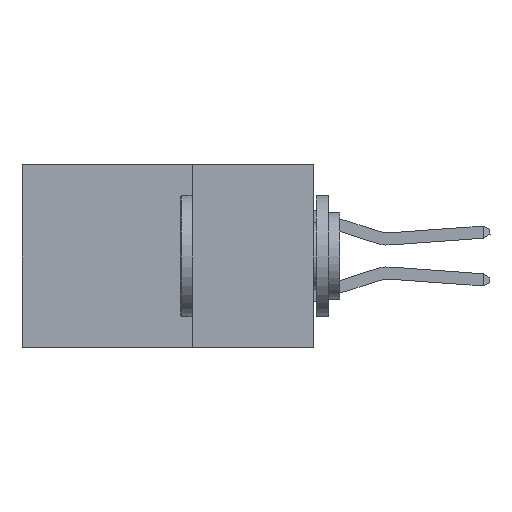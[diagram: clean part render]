
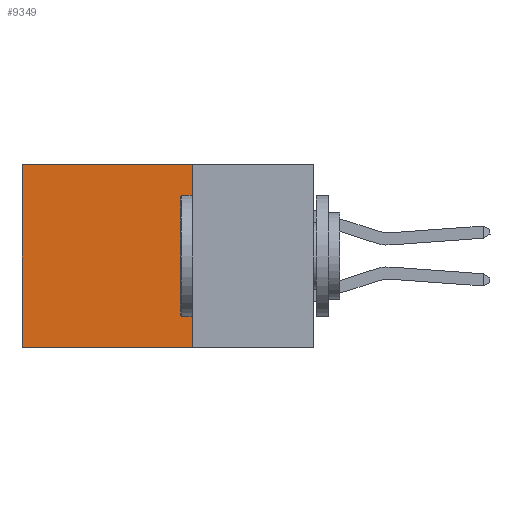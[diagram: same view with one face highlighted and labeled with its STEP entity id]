
A CAD part, left-side view. The second image highlights one B-rep face of the part: STEP entity #9349.
In plain terms, the highlighted planar face has unit normal (-1, 0, 0).
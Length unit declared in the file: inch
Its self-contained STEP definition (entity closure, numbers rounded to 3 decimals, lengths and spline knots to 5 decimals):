
#368 = VERTEX_POINT ( 'NONE', #6260 ) ;
#811 = DIRECTION ( 'NONE',  ( 0., 1., 0. ) ) ;
#1485 = CARTESIAN_POINT ( 'NONE',  ( 0.2875, 0.6, -0.375 ) ) ;
#2697 = AXIS2_PLACEMENT_3D ( 'NONE', #14191, #8348, #5224 ) ;
#2864 = VECTOR ( 'NONE', #811, 39.37008 ) ;
#2972 = ORIENTED_EDGE ( 'NONE', *, *, #7686, .F. ) ;
#3616 = CARTESIAN_POINT ( 'NONE',  ( 0.2875, 0.6, 0. ) ) ;
#3861 = DIRECTION ( 'NONE',  ( 0., 1., 0. ) ) ;
#5224 = DIRECTION ( 'NONE',  ( 0., 0., -1. ) ) ;
#5724 = CARTESIAN_POINT ( 'NONE',  ( 0.2875, 0.25, -0.375 ) ) ;
#6260 = CARTESIAN_POINT ( 'NONE',  ( 0.2875, 0.6, -0.375 ) ) ;
#6409 = CARTESIAN_POINT ( 'NONE',  ( 0.2875, 0.25, -0.375 ) ) ;
#7025 = EDGE_CURVE ( 'NONE', #10077, #368, #10886, .T. ) ;
#7678 = VERTEX_POINT ( 'NONE', #15529 ) ;
#7686 = EDGE_CURVE ( 'NONE', #7678, #10077, #18192, .T. ) ;
#8348 = DIRECTION ( 'NONE',  ( 1., 0., 0. ) ) ;
#9180 = VECTOR ( 'NONE', #10527, 39.37008 ) ;
#9344 = EDGE_CURVE ( 'NONE', #7678, #10639, #14052, .T. ) ;
#9349 = ADVANCED_FACE ( 'NONE', ( #13579 ), #19061, .F. ) ;
#9946 = EDGE_LOOP ( 'NONE', ( #19256, #12822, #2972, #17347 ) ) ;
#10061 = VECTOR ( 'NONE', #3861, 39.37008 ) ;
#10077 = VERTEX_POINT ( 'NONE', #5724 ) ;
#10527 = DIRECTION ( 'NONE',  ( 0., 0., -1. ) ) ;
#10639 = VERTEX_POINT ( 'NONE', #3616 ) ;
#10886 = LINE ( 'NONE', #14445, #2864 ) ;
#12457 = LINE ( 'NONE', #1485, #9180 ) ;
#12822 = ORIENTED_EDGE ( 'NONE', *, *, #7025, .F. ) ;
#13579 = FACE_OUTER_BOUND ( 'NONE', #9946, .T. ) ;
#14002 = DIRECTION ( 'NONE',  ( 0., 0., -1. ) ) ;
#14052 = LINE ( 'NONE', #18994, #10061 ) ;
#14120 = VECTOR ( 'NONE', #14002, 39.37008 ) ;
#14191 = CARTESIAN_POINT ( 'NONE',  ( 0.2875, 0.25, -0.375 ) ) ;
#14445 = CARTESIAN_POINT ( 'NONE',  ( 0.2875, 0.25, -0.375 ) ) ;
#15529 = CARTESIAN_POINT ( 'NONE',  ( 0.2875, 0.25, 0. ) ) ;
#17347 = ORIENTED_EDGE ( 'NONE', *, *, #9344, .T. ) ;
#18192 = LINE ( 'NONE', #6409, #14120 ) ;
#18994 = CARTESIAN_POINT ( 'NONE',  ( 0.2875, 0.25, 0. ) ) ;
#19061 = PLANE ( 'NONE',  #2697 ) ;
#19256 = ORIENTED_EDGE ( 'NONE', *, *, #19458, .T. ) ;
#19458 = EDGE_CURVE ( 'NONE', #10639, #368, #12457, .T. ) ;
